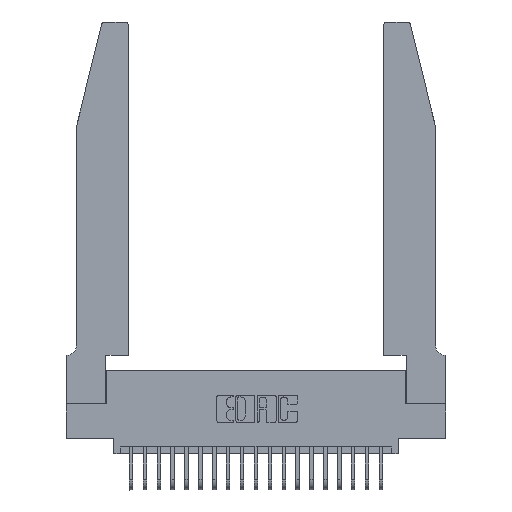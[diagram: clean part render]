
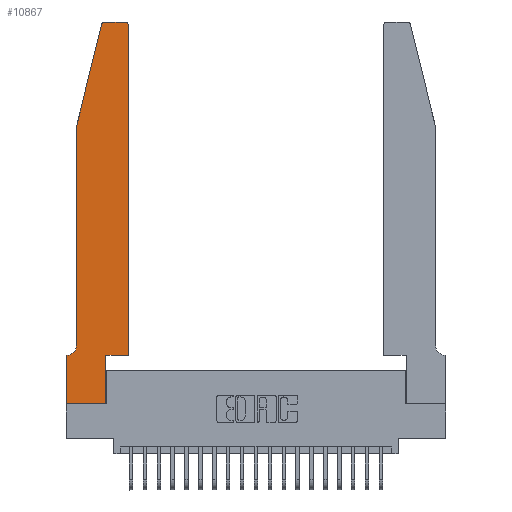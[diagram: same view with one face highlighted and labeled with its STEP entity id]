
A CAD part, top view. The second image highlights one B-rep face of the part: STEP entity #10867.
In plain terms, the highlighted planar face has unit normal (0, 0, 1).
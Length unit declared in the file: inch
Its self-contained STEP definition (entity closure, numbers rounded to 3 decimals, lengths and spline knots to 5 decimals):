
#179 = DIRECTION ( 'NONE',  ( 0., 0., -1. ) ) ;
#209 = LINE ( 'NONE', #9832, #801 ) ;
#681 = CARTESIAN_POINT ( 'NONE',  ( 0., 0.35, 0.37 ) ) ;
#801 = VECTOR ( 'NONE', #11535, 39.37008 ) ;
#916 = LINE ( 'NONE', #8976, #6214 ) ;
#1116 = CARTESIAN_POINT ( 'NONE',  ( 0.2605, 2.75, 0.37 ) ) ;
#1494 = ORIENTED_EDGE ( 'NONE', *, *, #18706, .T. ) ;
#1499 = VERTEX_POINT ( 'NONE', #11886 ) ;
#1503 = DIRECTION ( 'NONE',  ( 0., 1., 0. ) ) ;
#1796 = DIRECTION ( 'NONE',  ( 0., -1., 0. ) ) ;
#2277 = CARTESIAN_POINT ( 'NONE',  ( 0., 0., 0.37 ) ) ;
#2487 = DIRECTION ( 'NONE',  ( 0., 0., 1. ) ) ;
#2541 = CARTESIAN_POINT ( 'NONE',  ( 0.284, 2.72, 0.37 ) ) ;
#2567 = VECTOR ( 'NONE', #13635, 39.37008 ) ;
#2681 = EDGE_CURVE ( 'NONE', #17525, #16233, #4104, .T. ) ;
#3015 = CARTESIAN_POINT ( 'NONE',  ( 0.0755, 2., 0.37 ) ) ;
#3817 = VECTOR ( 'NONE', #9306, 39.37008 ) ;
#3956 = ORIENTED_EDGE ( 'NONE', *, *, #20012, .T. ) ;
#4104 = LINE ( 'NONE', #20055, #12808 ) ;
#4337 = DIRECTION ( 'NONE',  ( 1., 0., 0. ) ) ;
#4553 = ORIENTED_EDGE ( 'NONE', *, *, #6518, .T. ) ;
#4625 = CIRCLE ( 'NONE', #17448, 0.03 ) ;
#5508 = LINE ( 'NONE', #2277, #3817 ) ;
#5542 = EDGE_LOOP ( 'NONE', ( #19941, #19545, #4553, #13284, #6264, #14839, #14415, #3956, #6181, #19861, #7032, #1494 ) ) ;
#5570 = EDGE_CURVE ( 'NONE', #9100, #10429, #16416, .T. ) ;
#5775 = VERTEX_POINT ( 'NONE', #17903 ) ;
#6046 = AXIS2_PLACEMENT_3D ( 'NONE', #681, #2487, #14611 ) ;
#6147 = EDGE_CURVE ( 'NONE', #10429, #9556, #916, .T. ) ;
#6181 = ORIENTED_EDGE ( 'NONE', *, *, #5570, .T. ) ;
#6214 = VECTOR ( 'NONE', #17367, 39.37008 ) ;
#6264 = ORIENTED_EDGE ( 'NONE', *, *, #6820, .T. ) ;
#6455 = CARTESIAN_POINT ( 'NONE',  ( 0.4205, 2.72, 0.37 ) ) ;
#6518 = EDGE_CURVE ( 'NONE', #8108, #16391, #12418, .T. ) ;
#6738 = LINE ( 'NONE', #20368, #2567 ) ;
#6820 = EDGE_CURVE ( 'NONE', #6988, #17525, #11616, .T. ) ;
#6988 = VERTEX_POINT ( 'NONE', #14532 ) ;
#7032 = ORIENTED_EDGE ( 'NONE', *, *, #10957, .T. ) ;
#7424 = CARTESIAN_POINT ( 'NONE',  ( 0.4505, 0.35, 0.37 ) ) ;
#7823 = VECTOR ( 'NONE', #13448, 39.37008 ) ;
#8108 = VERTEX_POINT ( 'NONE', #18192 ) ;
#8224 = DIRECTION ( 'NONE',  ( 1., 0., 0. ) ) ;
#8259 = CARTESIAN_POINT ( 'NONE',  ( 0.284, 2.75, 0.37 ) ) ;
#8976 = CARTESIAN_POINT ( 'NONE',  ( 0.4505, 0.35, 0.37 ) ) ;
#8978 = VECTOR ( 'NONE', #1503, 39.37008 ) ;
#9100 = VERTEX_POINT ( 'NONE', #9173 ) ;
#9173 = CARTESIAN_POINT ( 'NONE',  ( 0.2865, 0., 0.37 ) ) ;
#9306 = DIRECTION ( 'NONE',  ( 0., -1., 0. ) ) ;
#9556 = VERTEX_POINT ( 'NONE', #7424 ) ;
#9832 = CARTESIAN_POINT ( 'NONE',  ( 0.4505, 0.35, 0.37 ) ) ;
#9942 = DIRECTION ( 'NONE',  ( -1., 0., 0. ) ) ;
#10429 = VERTEX_POINT ( 'NONE', #16710 ) ;
#10598 = AXIS2_PLACEMENT_3D ( 'NONE', #10793, #179, #12492 ) ;
#10627 = EDGE_CURVE ( 'NONE', #16391, #6988, #20540, .T. ) ;
#10793 = CARTESIAN_POINT ( 'NONE',  ( 0.0055, 0.42, 0.37 ) ) ;
#10828 = CARTESIAN_POINT ( 'NONE',  ( 0.0055, 0.35, 0.37 ) ) ;
#10867 = ADVANCED_FACE ( 'NONE', ( #16282 ), #11244, .T. ) ;
#10957 = EDGE_CURVE ( 'NONE', #9556, #1499, #209, .T. ) ;
#11244 = PLANE ( 'NONE',  #6046 ) ;
#11535 = DIRECTION ( 'NONE',  ( 0., 1., 0. ) ) ;
#11555 = VECTOR ( 'NONE', #1796, 39.37008 ) ;
#11616 = CIRCLE ( 'NONE', #10598, 0.07 ) ;
#11624 = VERTEX_POINT ( 'NONE', #8259 ) ;
#11793 = CARTESIAN_POINT ( 'NONE',  ( 0., 0., 0.37 ) ) ;
#11886 = CARTESIAN_POINT ( 'NONE',  ( 0.4505, 2.72, 0.37 ) ) ;
#12418 = LINE ( 'NONE', #3015, #7823 ) ;
#12492 = DIRECTION ( 'NONE',  ( -1., 0., 0. ) ) ;
#12572 = EDGE_CURVE ( 'NONE', #16233, #14127, #5508, .T. ) ;
#12808 = VECTOR ( 'NONE', #21633, 39.37008 ) ;
#13092 = VECTOR ( 'NONE', #9942, 39.37008 ) ;
#13284 = ORIENTED_EDGE ( 'NONE', *, *, #10627, .T. ) ;
#13448 = DIRECTION ( 'NONE',  ( -0.239, -0.971, 0. ) ) ;
#13624 = LINE ( 'NONE', #1116, #13092 ) ;
#13635 = DIRECTION ( 'NONE',  ( 1., 0., 0. ) ) ;
#13975 = CARTESIAN_POINT ( 'NONE',  ( 0.0755, 2., 0.37 ) ) ;
#14018 = CIRCLE ( 'NONE', #14202, 0.03 ) ;
#14127 = VERTEX_POINT ( 'NONE', #11793 ) ;
#14202 = AXIS2_PLACEMENT_3D ( 'NONE', #6455, #18420, #8224 ) ;
#14415 = ORIENTED_EDGE ( 'NONE', *, *, #12572, .T. ) ;
#14532 = CARTESIAN_POINT ( 'NONE',  ( 0.0755, 0.42, 0.37 ) ) ;
#14611 = DIRECTION ( 'NONE',  ( 1., 0., 0. ) ) ;
#14672 = DIRECTION ( 'NONE',  ( 0., 0., 1. ) ) ;
#14839 = ORIENTED_EDGE ( 'NONE', *, *, #2681, .T. ) ;
#15968 = EDGE_CURVE ( 'NONE', #5775, #11624, #13624, .T. ) ;
#16233 = VERTEX_POINT ( 'NONE', #19107 ) ;
#16282 = FACE_OUTER_BOUND ( 'NONE', #5542, .T. ) ;
#16391 = VERTEX_POINT ( 'NONE', #21132 ) ;
#16416 = LINE ( 'NONE', #18818, #8978 ) ;
#16710 = CARTESIAN_POINT ( 'NONE',  ( 0.2865, 0.35, 0.37 ) ) ;
#17125 = EDGE_CURVE ( 'NONE', #11624, #8108, #4625, .T. ) ;
#17367 = DIRECTION ( 'NONE',  ( 1., 0., 0. ) ) ;
#17448 = AXIS2_PLACEMENT_3D ( 'NONE', #2541, #14672, #4337 ) ;
#17525 = VERTEX_POINT ( 'NONE', #10828 ) ;
#17903 = CARTESIAN_POINT ( 'NONE',  ( 0.4205, 2.75, 0.37 ) ) ;
#18192 = CARTESIAN_POINT ( 'NONE',  ( 0.25487, 2.72718, 0.37 ) ) ;
#18420 = DIRECTION ( 'NONE',  ( 0., 0., 1. ) ) ;
#18706 = EDGE_CURVE ( 'NONE', #1499, #5775, #14018, .T. ) ;
#18818 = CARTESIAN_POINT ( 'NONE',  ( 0.2865, 0.35, 0.37 ) ) ;
#19107 = CARTESIAN_POINT ( 'NONE',  ( 0., 0.35, 0.37 ) ) ;
#19545 = ORIENTED_EDGE ( 'NONE', *, *, #17125, .T. ) ;
#19861 = ORIENTED_EDGE ( 'NONE', *, *, #6147, .T. ) ;
#19941 = ORIENTED_EDGE ( 'NONE', *, *, #15968, .T. ) ;
#20012 = EDGE_CURVE ( 'NONE', #14127, #9100, #6738, .T. ) ;
#20055 = CARTESIAN_POINT ( 'NONE',  ( 0.0755, 0.35, 0.37 ) ) ;
#20368 = CARTESIAN_POINT ( 'NONE',  ( 0., 0., 0.37 ) ) ;
#20540 = LINE ( 'NONE', #13975, #11555 ) ;
#21132 = CARTESIAN_POINT ( 'NONE',  ( 0.0755, 2., 0.37 ) ) ;
#21633 = DIRECTION ( 'NONE',  ( -1., 0., 0. ) ) ;
